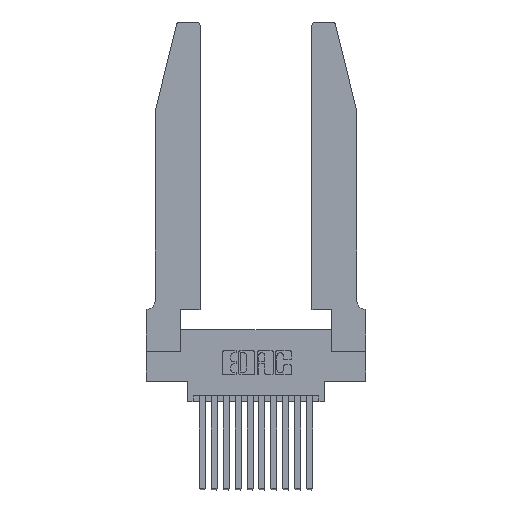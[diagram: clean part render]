
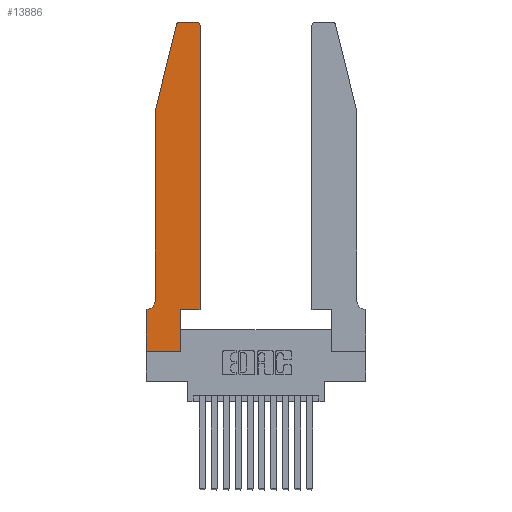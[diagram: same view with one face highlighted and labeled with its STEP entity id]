
A CAD part, top view. The second image highlights one B-rep face of the part: STEP entity #13886.
In plain terms, the highlighted planar face has unit normal (0, 0, 1).
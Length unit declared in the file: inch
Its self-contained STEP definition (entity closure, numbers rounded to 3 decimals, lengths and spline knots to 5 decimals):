
#93 = CARTESIAN_POINT ( 'NONE',  ( 0., 0.35, 0.37 ) ) ;
#443 = VERTEX_POINT ( 'NONE', #14763 ) ;
#501 = VECTOR ( 'NONE', #1294, 39.37008 ) ;
#601 = CARTESIAN_POINT ( 'NONE',  ( 0.4505, 0.35, 0.37 ) ) ;
#724 = CARTESIAN_POINT ( 'NONE',  ( 0.0755, 2., 0.37 ) ) ;
#970 = ORIENTED_EDGE ( 'NONE', *, *, #1272, .T. ) ;
#1046 = ORIENTED_EDGE ( 'NONE', *, *, #4048, .T. ) ;
#1185 = ORIENTED_EDGE ( 'NONE', *, *, #15676, .T. ) ;
#1272 = EDGE_CURVE ( 'NONE', #13829, #5823, #15860, .T. ) ;
#1294 = DIRECTION ( 'NONE',  ( 1., 0., 0. ) ) ;
#1313 = CARTESIAN_POINT ( 'NONE',  ( 0.25487, 2.72718, 0.37 ) ) ;
#1347 = DIRECTION ( 'NONE',  ( 0., 1., 0. ) ) ;
#1447 = ORIENTED_EDGE ( 'NONE', *, *, #13481, .T. ) ;
#1482 = DIRECTION ( 'NONE',  ( 0., 0., 1. ) ) ;
#1501 = CARTESIAN_POINT ( 'NONE',  ( 0., 0., 0.37 ) ) ;
#1502 = ORIENTED_EDGE ( 'NONE', *, *, #5322, .T. ) ;
#1562 = VERTEX_POINT ( 'NONE', #14243 ) ;
#1750 = ORIENTED_EDGE ( 'NONE', *, *, #12203, .T. ) ;
#1865 = ORIENTED_EDGE ( 'NONE', *, *, #16852, .T. ) ;
#1964 = CARTESIAN_POINT ( 'NONE',  ( 0.0055, 0.35, 0.37 ) ) ;
#2114 = DIRECTION ( 'NONE',  ( 0., -1., 0. ) ) ;
#2297 = VECTOR ( 'NONE', #1347, 39.37008 ) ;
#2359 = ORIENTED_EDGE ( 'NONE', *, *, #13282, .T. ) ;
#2407 = ORIENTED_EDGE ( 'NONE', *, *, #12372, .T. ) ;
#2650 = CARTESIAN_POINT ( 'NONE',  ( 0.0755, 0.42, 0.37 ) ) ;
#2897 = ORIENTED_EDGE ( 'NONE', *, *, #4387, .T. ) ;
#2910 = DIRECTION ( 'NONE',  ( 1., 0., 0. ) ) ;
#4016 = AXIS2_PLACEMENT_3D ( 'NONE', #7430, #16249, #8723 ) ;
#4048 = EDGE_CURVE ( 'NONE', #1562, #8776, #6424, .T. ) ;
#4060 = VECTOR ( 'NONE', #14653, 39.37008 ) ;
#4121 = LINE ( 'NONE', #10582, #501 ) ;
#4155 = VECTOR ( 'NONE', #2114, 39.37008 ) ;
#4293 = VERTEX_POINT ( 'NONE', #6779 ) ;
#4316 = DIRECTION ( 'NONE',  ( 0., 0., 1. ) ) ;
#4344 = CARTESIAN_POINT ( 'NONE',  ( 0.4505, 0.35, 0.37 ) ) ;
#4387 = EDGE_CURVE ( 'NONE', #8776, #13829, #8504, .T. ) ;
#4960 = VERTEX_POINT ( 'NONE', #601 ) ;
#4969 = CARTESIAN_POINT ( 'NONE',  ( 0.0755, 2., 0.37 ) ) ;
#5023 = DIRECTION ( 'NONE',  ( -1., 0., 0. ) ) ;
#5096 = ORIENTED_EDGE ( 'NONE', *, *, #6345, .T. ) ;
#5260 = AXIS2_PLACEMENT_3D ( 'NONE', #14455, #6825, #15725 ) ;
#5317 = VERTEX_POINT ( 'NONE', #2650 ) ;
#5322 = EDGE_CURVE ( 'NONE', #443, #6754, #6607, .T. ) ;
#5375 = CARTESIAN_POINT ( 'NONE',  ( 0.2865, 0.35, 0.37 ) ) ;
#5492 = LINE ( 'NONE', #1501, #15309 ) ;
#5743 = ORIENTED_EDGE ( 'NONE', *, *, #15919, .T. ) ;
#5785 = VECTOR ( 'NONE', #11829, 39.37008 ) ;
#5823 = VERTEX_POINT ( 'NONE', #4969 ) ;
#6094 = DIRECTION ( 'NONE',  ( -1., 0., 0. ) ) ;
#6345 = EDGE_CURVE ( 'NONE', #8456, #4293, #12717, .T. ) ;
#6424 = LINE ( 'NONE', #11502, #9517 ) ;
#6607 = LINE ( 'NONE', #10590, #5785 ) ;
#6754 = VERTEX_POINT ( 'NONE', #12533 ) ;
#6779 = CARTESIAN_POINT ( 'NONE',  ( 0.2865, 0.35, 0.37 ) ) ;
#6825 = DIRECTION ( 'NONE',  ( 0., 0., -1. ) ) ;
#7430 = CARTESIAN_POINT ( 'NONE',  ( 0.4205, 2.72, 0.37 ) ) ;
#7638 = LINE ( 'NONE', #4344, #4060 ) ;
#7941 = CARTESIAN_POINT ( 'NONE',  ( 0.284, 2.75, 0.37 ) ) ;
#7994 = DIRECTION ( 'NONE',  ( -0.239, -0.971, 0. ) ) ;
#8221 = PLANE ( 'NONE',  #10715 ) ;
#8456 = VERTEX_POINT ( 'NONE', #15673 ) ;
#8504 = CIRCLE ( 'NONE', #16166, 0.03 ) ;
#8723 = DIRECTION ( 'NONE',  ( 1., 0., 0. ) ) ;
#8776 = VERTEX_POINT ( 'NONE', #7941 ) ;
#9517 = VECTOR ( 'NONE', #5023, 39.37008 ) ;
#10000 = FACE_OUTER_BOUND ( 'NONE', #12344, .T. ) ;
#10244 = CARTESIAN_POINT ( 'NONE',  ( 0.0755, 2., 0.37 ) ) ;
#10514 = VERTEX_POINT ( 'NONE', #13024 ) ;
#10582 = CARTESIAN_POINT ( 'NONE',  ( 0.4505, 0.35, 0.37 ) ) ;
#10590 = CARTESIAN_POINT ( 'NONE',  ( 0., 0., 0.37 ) ) ;
#10715 = AXIS2_PLACEMENT_3D ( 'NONE', #93, #1482, #10756 ) ;
#10756 = DIRECTION ( 'NONE',  ( 1., 0., 0. ) ) ;
#11502 = CARTESIAN_POINT ( 'NONE',  ( 0.2605, 2.75, 0.37 ) ) ;
#11829 = DIRECTION ( 'NONE',  ( 0., -1., 0. ) ) ;
#11970 = VECTOR ( 'NONE', #6094, 39.37008 ) ;
#12083 = CARTESIAN_POINT ( 'NONE',  ( 0.284, 2.72, 0.37 ) ) ;
#12203 = EDGE_CURVE ( 'NONE', #4960, #10514, #7638, .T. ) ;
#12344 = EDGE_LOOP ( 'NONE', ( #1046, #2897, #970, #5743, #1185, #2407, #1502, #2359, #5096, #1865, #1750, #1447 ) ) ;
#12372 = EDGE_CURVE ( 'NONE', #16493, #443, #15342, .T. ) ;
#12533 = CARTESIAN_POINT ( 'NONE',  ( 0., 0., 0.37 ) ) ;
#12538 = CIRCLE ( 'NONE', #4016, 0.03 ) ;
#12717 = LINE ( 'NONE', #5375, #2297 ) ;
#13024 = CARTESIAN_POINT ( 'NONE',  ( 0.4505, 2.72, 0.37 ) ) ;
#13282 = EDGE_CURVE ( 'NONE', #6754, #8456, #5492, .T. ) ;
#13384 = DIRECTION ( 'NONE',  ( 1., 0., 0. ) ) ;
#13481 = EDGE_CURVE ( 'NONE', #10514, #1562, #12538, .T. ) ;
#13797 = CARTESIAN_POINT ( 'NONE',  ( 0.0755, 0.35, 0.37 ) ) ;
#13829 = VERTEX_POINT ( 'NONE', #1313 ) ;
#13886 = ADVANCED_FACE ( 'NONE', ( #10000 ), #8221, .T. ) ;
#14243 = CARTESIAN_POINT ( 'NONE',  ( 0.4205, 2.75, 0.37 ) ) ;
#14435 = CIRCLE ( 'NONE', #5260, 0.07 ) ;
#14454 = LINE ( 'NONE', #724, #4155 ) ;
#14455 = CARTESIAN_POINT ( 'NONE',  ( 0.0055, 0.42, 0.37 ) ) ;
#14653 = DIRECTION ( 'NONE',  ( 0., 1., 0. ) ) ;
#14763 = CARTESIAN_POINT ( 'NONE',  ( 0., 0.35, 0.37 ) ) ;
#15309 = VECTOR ( 'NONE', #2910, 39.37008 ) ;
#15342 = LINE ( 'NONE', #13797, #11970 ) ;
#15465 = VECTOR ( 'NONE', #7994, 39.37008 ) ;
#15673 = CARTESIAN_POINT ( 'NONE',  ( 0.2865, 0., 0.37 ) ) ;
#15676 = EDGE_CURVE ( 'NONE', #5317, #16493, #14435, .T. ) ;
#15725 = DIRECTION ( 'NONE',  ( -1., 0., 0. ) ) ;
#15860 = LINE ( 'NONE', #10244, #15465 ) ;
#15919 = EDGE_CURVE ( 'NONE', #5823, #5317, #14454, .T. ) ;
#16166 = AXIS2_PLACEMENT_3D ( 'NONE', #12083, #4316, #13384 ) ;
#16249 = DIRECTION ( 'NONE',  ( 0., 0., 1. ) ) ;
#16493 = VERTEX_POINT ( 'NONE', #1964 ) ;
#16852 = EDGE_CURVE ( 'NONE', #4293, #4960, #4121, .T. ) ;
